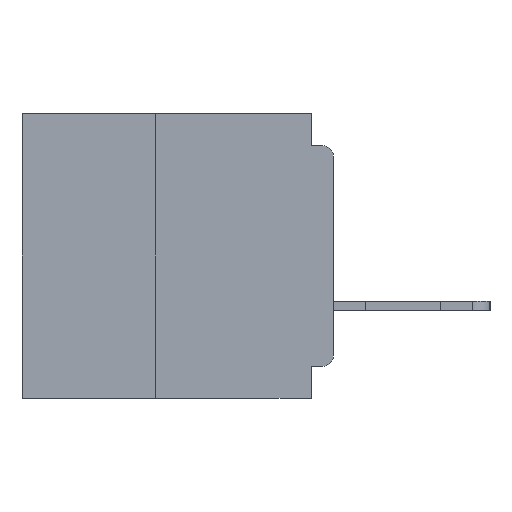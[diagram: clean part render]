
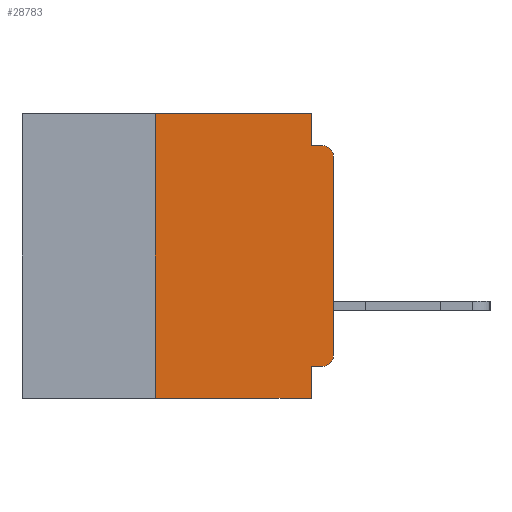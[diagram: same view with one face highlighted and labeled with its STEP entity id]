
A CAD part, left-side view. The second image highlights one B-rep face of the part: STEP entity #28783.
In plain terms, the highlighted planar face has unit normal (-1, 0, 0).
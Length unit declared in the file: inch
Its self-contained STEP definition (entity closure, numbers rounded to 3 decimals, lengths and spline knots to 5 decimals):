
#218 = DIRECTION ( 'NONE',  ( 0., 0., 1. ) ) ;
#470 = LINE ( 'NONE', #21458, #8976 ) ;
#614 = DIRECTION ( 'NONE',  ( 0., 0., -1. ) ) ;
#849 = VERTEX_POINT ( 'NONE', #29142 ) ;
#1301 = LINE ( 'NONE', #43434, #38588 ) ;
#1394 = DIRECTION ( 'NONE',  ( 0., -1., 0. ) ) ;
#1840 = VERTEX_POINT ( 'NONE', #33519 ) ;
#3499 = DIRECTION ( 'NONE',  ( 0., 0., -1. ) ) ;
#4299 = LINE ( 'NONE', #35323, #31941 ) ;
#4896 = LINE ( 'NONE', #33357, #31379 ) ;
#5294 = ORIENTED_EDGE ( 'NONE', *, *, #41646, .T. ) ;
#5630 = DIRECTION ( 'NONE',  ( -1., 0., 0. ) ) ;
#6920 = EDGE_CURVE ( 'NONE', #8216, #34855, #1301, .T. ) ;
#7791 = VERTEX_POINT ( 'NONE', #23193 ) ;
#8216 = VERTEX_POINT ( 'NONE', #33155 ) ;
#8263 = LINE ( 'NONE', #38203, #17783 ) ;
#8781 = VERTEX_POINT ( 'NONE', #21983 ) ;
#8976 = VECTOR ( 'NONE', #3499, 39.37008 ) ;
#9321 = EDGE_CURVE ( 'NONE', #33460, #849, #470, .T. ) ;
#9883 = ORIENTED_EDGE ( 'NONE', *, *, #39250, .F. ) ;
#10203 = ORIENTED_EDGE ( 'NONE', *, *, #26577, .F. ) ;
#12111 = CIRCLE ( 'NONE', #27166, 0.015 ) ;
#13604 = DIRECTION ( 'NONE',  ( 0., 1., 0. ) ) ;
#16518 = DIRECTION ( 'NONE',  ( 0., -1., 0. ) ) ;
#16637 = LINE ( 'NONE', #39282, #27397 ) ;
#17104 = LINE ( 'NONE', #23013, #35276 ) ;
#17783 = VECTOR ( 'NONE', #27253, 39.37008 ) ;
#17977 = ORIENTED_EDGE ( 'NONE', *, *, #9321, .F. ) ;
#18242 = LINE ( 'NONE', #20029, #35258 ) ;
#18887 = CARTESIAN_POINT ( 'NONE',  ( 0., 0.031, 0. ) ) ;
#19296 = DIRECTION ( 'NONE',  ( -1., 0., 0. ) ) ;
#20029 = CARTESIAN_POINT ( 'NONE',  ( 0., 0.437, -0.4 ) ) ;
#20869 = CARTESIAN_POINT ( 'NONE',  ( 0., 0.25, 0. ) ) ;
#21458 = CARTESIAN_POINT ( 'NONE',  ( 0., 0.031, 0. ) ) ;
#21486 = CARTESIAN_POINT ( 'NONE',  ( 0., 0.031, -0.4 ) ) ;
#21983 = CARTESIAN_POINT ( 'NONE',  ( 0., 0.015, -0.045 ) ) ;
#22243 = DIRECTION ( 'NONE',  ( 1., 0., 0. ) ) ;
#23013 = CARTESIAN_POINT ( 'NONE',  ( 0., 0.437, 0. ) ) ;
#23193 = CARTESIAN_POINT ( 'NONE',  ( 0., 0., -0.34 ) ) ;
#23960 = ORIENTED_EDGE ( 'NONE', *, *, #6920, .F. ) ;
#25232 = AXIS2_PLACEMENT_3D ( 'NONE', #33029, #22243, #614 ) ;
#25838 = EDGE_LOOP ( 'NONE', ( #42451, #29911, #10203, #17977, #34371, #23960, #5294, #9883, #41652, #26195 ) ) ;
#26002 = VERTEX_POINT ( 'NONE', #21486 ) ;
#26195 = ORIENTED_EDGE ( 'NONE', *, *, #27454, .T. ) ;
#26577 = EDGE_CURVE ( 'NONE', #849, #8781, #16637, .T. ) ;
#27166 = AXIS2_PLACEMENT_3D ( 'NONE', #40915, #19296, #44503 ) ;
#27177 = CARTESIAN_POINT ( 'NONE',  ( 0., 0.015, -0.34 ) ) ;
#27253 = DIRECTION ( 'NONE',  ( 0., 0., -1. ) ) ;
#27284 = AXIS2_PLACEMENT_3D ( 'NONE', #27177, #5630, #30844 ) ;
#27397 = VECTOR ( 'NONE', #46465, 39.37008 ) ;
#27454 = EDGE_CURVE ( 'NONE', #32308, #7791, #35857, .T. ) ;
#28783 = ADVANCED_FACE ( 'NONE', ( #36847 ), #43806, .F. ) ;
#29142 = CARTESIAN_POINT ( 'NONE',  ( 0., 0.031, -0.045 ) ) ;
#29614 = CARTESIAN_POINT ( 'NONE',  ( 0., 0., -0.06 ) ) ;
#29911 = ORIENTED_EDGE ( 'NONE', *, *, #32351, .T. ) ;
#30844 = DIRECTION ( 'NONE',  ( 0., 0., -1. ) ) ;
#31379 = VECTOR ( 'NONE', #41181, 39.37008 ) ;
#31941 = VECTOR ( 'NONE', #13604, 39.37008 ) ;
#32308 = VERTEX_POINT ( 'NONE', #44191 ) ;
#32351 = EDGE_CURVE ( 'NONE', #37894, #8781, #12111, .T. ) ;
#33029 = CARTESIAN_POINT ( 'NONE',  ( 0., 0.437, 0. ) ) ;
#33155 = CARTESIAN_POINT ( 'NONE',  ( 0., 0.25, -0.4 ) ) ;
#33357 = CARTESIAN_POINT ( 'NONE',  ( 0., 0., 0. ) ) ;
#33460 = VERTEX_POINT ( 'NONE', #18887 ) ;
#33519 = CARTESIAN_POINT ( 'NONE',  ( 0., 0.031, -0.355 ) ) ;
#34371 = ORIENTED_EDGE ( 'NONE', *, *, #40316, .F. ) ;
#34855 = VERTEX_POINT ( 'NONE', #20869 ) ;
#35258 = VECTOR ( 'NONE', #16518, 39.37008 ) ;
#35276 = VECTOR ( 'NONE', #1394, 39.37008 ) ;
#35323 = CARTESIAN_POINT ( 'NONE',  ( 0., 0., -0.355 ) ) ;
#35857 = CIRCLE ( 'NONE', #27284, 0.015 ) ;
#36847 = FACE_OUTER_BOUND ( 'NONE', #25838, .T. ) ;
#37894 = VERTEX_POINT ( 'NONE', #29614 ) ;
#38203 = CARTESIAN_POINT ( 'NONE',  ( 0., 0.031, -0.4 ) ) ;
#38588 = VECTOR ( 'NONE', #218, 39.37008 ) ;
#39250 = EDGE_CURVE ( 'NONE', #1840, #26002, #8263, .T. ) ;
#39282 = CARTESIAN_POINT ( 'NONE',  ( 0., 0., -0.045 ) ) ;
#40316 = EDGE_CURVE ( 'NONE', #34855, #33460, #17104, .T. ) ;
#40915 = CARTESIAN_POINT ( 'NONE',  ( 0., 0.015, -0.06 ) ) ;
#41181 = DIRECTION ( 'NONE',  ( 0., 0., 1. ) ) ;
#41646 = EDGE_CURVE ( 'NONE', #8216, #26002, #18242, .T. ) ;
#41652 = ORIENTED_EDGE ( 'NONE', *, *, #46779, .F. ) ;
#42451 = ORIENTED_EDGE ( 'NONE', *, *, #45883, .T. ) ;
#43434 = CARTESIAN_POINT ( 'NONE',  ( 0., 0.25, -0.4 ) ) ;
#43806 = PLANE ( 'NONE',  #25232 ) ;
#44191 = CARTESIAN_POINT ( 'NONE',  ( 0., 0.015, -0.355 ) ) ;
#44503 = DIRECTION ( 'NONE',  ( 0., 0., -1. ) ) ;
#45883 = EDGE_CURVE ( 'NONE', #7791, #37894, #4896, .T. ) ;
#46465 = DIRECTION ( 'NONE',  ( 0., -1., 0. ) ) ;
#46779 = EDGE_CURVE ( 'NONE', #32308, #1840, #4299, .T. ) ;
